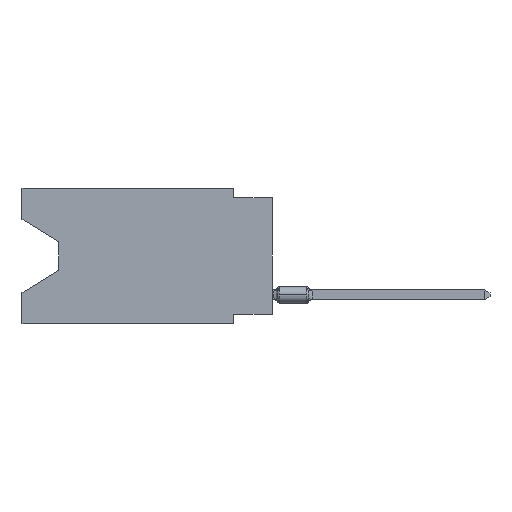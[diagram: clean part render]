
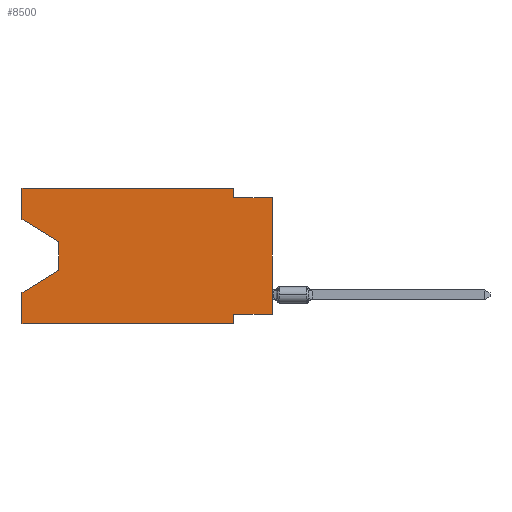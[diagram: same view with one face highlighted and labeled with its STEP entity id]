
A CAD part, left-side view. The second image highlights one B-rep face of the part: STEP entity #8500.
In plain terms, the highlighted planar face has unit normal (-1, 0, 0).
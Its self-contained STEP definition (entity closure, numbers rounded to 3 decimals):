
#78 = CARTESIAN_POINT ( 'NONE',  ( 0., 16.383, 0. ) ) ;
#345 = VERTEX_POINT ( 'NONE', #19564 ) ;
#853 = VERTEX_POINT ( 'NONE', #15511 ) ;
#1800 = EDGE_LOOP ( 'NONE', ( #27748, #20072, #8516, #16104, #6774, #10300, #17275, #5367, #20971, #21598, #28612, #13708 ) ) ;
#1977 = DIRECTION ( 'NONE',  ( 0., 0., -1. ) ) ;
#2008 = VECTOR ( 'NONE', #23691, 1000. ) ;
#3251 = VECTOR ( 'NONE', #20385, 1000. ) ;
#3297 = AXIS2_PLACEMENT_3D ( 'NONE', #5024, #9683, #28205 ) ;
#3729 = LINE ( 'NONE', #27179, #3251 ) ;
#4278 = CARTESIAN_POINT ( 'NONE',  ( 0., 2.54, -8.89 ) ) ;
#4324 = EDGE_CURVE ( 'NONE', #12260, #11319, #3729, .T. ) ;
#4360 = VERTEX_POINT ( 'NONE', #15780 ) ;
#4944 = DIRECTION ( 'NONE',  ( 0., 1., 0. ) ) ;
#5024 = CARTESIAN_POINT ( 'NONE',  ( 0., 16.383, 0. ) ) ;
#5367 = ORIENTED_EDGE ( 'NONE', *, *, #4324, .T. ) ;
#5720 = DIRECTION ( 'NONE',  ( 0., 0., -1. ) ) ;
#6063 = EDGE_CURVE ( 'NONE', #16725, #4360, #11096, .T. ) ;
#6774 = ORIENTED_EDGE ( 'NONE', *, *, #14630, .T. ) ;
#8034 = CARTESIAN_POINT ( 'NONE',  ( 0., 2.54, -8.255 ) ) ;
#8378 = CARTESIAN_POINT ( 'NONE',  ( 0., 0., -0.635 ) ) ;
#8500 = ADVANCED_FACE ( 'NONE', ( #30499 ), #18948, .F. ) ;
#8516 = ORIENTED_EDGE ( 'NONE', *, *, #21570, .T. ) ;
#8838 = VECTOR ( 'NONE', #27270, 1000. ) ;
#8897 = VERTEX_POINT ( 'NONE', #9176 ) ;
#8910 = EDGE_CURVE ( 'NONE', #28071, #29091, #14291, .T. ) ;
#8957 = LINE ( 'NONE', #27643, #15032 ) ;
#9023 = CARTESIAN_POINT ( 'NONE',  ( 0., 16.383, 0. ) ) ;
#9114 = EDGE_CURVE ( 'NONE', #345, #11319, #13198, .T. ) ;
#9176 = CARTESIAN_POINT ( 'NONE',  ( 0., 16.383, -6.852 ) ) ;
#9683 = DIRECTION ( 'NONE',  ( 1., 0., 0. ) ) ;
#10146 = EDGE_CURVE ( 'NONE', #12260, #16725, #20871, .T. ) ;
#10167 = LINE ( 'NONE', #19584, #15781 ) ;
#10300 = ORIENTED_EDGE ( 'NONE', *, *, #6063, .F. ) ;
#10469 = VECTOR ( 'NONE', #5720, 1000. ) ;
#10510 = CARTESIAN_POINT ( 'NONE',  ( 0., 13.97, -3.505 ) ) ;
#10679 = DIRECTION ( 'NONE',  ( 0., 0., -1. ) ) ;
#11096 = LINE ( 'NONE', #4278, #27362 ) ;
#11319 = VERTEX_POINT ( 'NONE', #28081 ) ;
#12260 = VERTEX_POINT ( 'NONE', #25673 ) ;
#12790 = LINE ( 'NONE', #18027, #8838 ) ;
#12844 = VECTOR ( 'NONE', #20445, 1000. ) ;
#12995 = LINE ( 'NONE', #10510, #14455 ) ;
#13198 = LINE ( 'NONE', #8378, #22211 ) ;
#13708 = ORIENTED_EDGE ( 'NONE', *, *, #8910, .F. ) ;
#13918 = CARTESIAN_POINT ( 'NONE',  ( 0., 13.97, -5.385 ) ) ;
#14291 = LINE ( 'NONE', #78, #2008 ) ;
#14455 = VECTOR ( 'NONE', #10679, 1000. ) ;
#14630 = EDGE_CURVE ( 'NONE', #15749, #4360, #10167, .T. ) ;
#14807 = VECTOR ( 'NONE', #4944, 1000. ) ;
#14820 = EDGE_CURVE ( 'NONE', #15749, #8897, #12790, .T. ) ;
#14952 = VECTOR ( 'NONE', #22784, 1000. ) ;
#15032 = VECTOR ( 'NONE', #29961, 1000. ) ;
#15265 = EDGE_CURVE ( 'NONE', #28071, #853, #26936, .T. ) ;
#15511 = CARTESIAN_POINT ( 'NONE',  ( 0., 13.97, -3.505 ) ) ;
#15749 = VERTEX_POINT ( 'NONE', #22546 ) ;
#15780 = CARTESIAN_POINT ( 'NONE',  ( 0., 2.54, -8.89 ) ) ;
#15781 = VECTOR ( 'NONE', #28996, 1000. ) ;
#16104 = ORIENTED_EDGE ( 'NONE', *, *, #14820, .F. ) ;
#16142 = CARTESIAN_POINT ( 'NONE',  ( 0., 16.383, 0. ) ) ;
#16725 = VERTEX_POINT ( 'NONE', #8034 ) ;
#17275 = ORIENTED_EDGE ( 'NONE', *, *, #10146, .F. ) ;
#17475 = CARTESIAN_POINT ( 'NONE',  ( 0., 2.54, 0. ) ) ;
#18027 = CARTESIAN_POINT ( 'NONE',  ( 0., 16.383, 0. ) ) ;
#18045 = VERTEX_POINT ( 'NONE', #24868 ) ;
#18857 = CARTESIAN_POINT ( 'NONE',  ( 0., 0., -8.255 ) ) ;
#18948 = PLANE ( 'NONE',  #3297 ) ;
#19516 = EDGE_CURVE ( 'NONE', #29091, #18045, #30167, .T. ) ;
#19564 = CARTESIAN_POINT ( 'NONE',  ( 0., 2.54, -0.635 ) ) ;
#19584 = CARTESIAN_POINT ( 'NONE',  ( 0., 16.383, -8.89 ) ) ;
#19981 = DIRECTION ( 'NONE',  ( 0., -1., 0. ) ) ;
#20072 = ORIENTED_EDGE ( 'NONE', *, *, #29893, .T. ) ;
#20385 = DIRECTION ( 'NONE',  ( 0., 0., 1. ) ) ;
#20445 = DIRECTION ( 'NONE',  ( 0., -0.855, -0.519 ) ) ;
#20871 = LINE ( 'NONE', #18857, #14807 ) ;
#20971 = ORIENTED_EDGE ( 'NONE', *, *, #9114, .F. ) ;
#21570 = EDGE_CURVE ( 'NONE', #30261, #8897, #8957, .T. ) ;
#21598 = ORIENTED_EDGE ( 'NONE', *, *, #29772, .F. ) ;
#22211 = VECTOR ( 'NONE', #19981, 1000. ) ;
#22546 = CARTESIAN_POINT ( 'NONE',  ( 0., 16.383, -8.89 ) ) ;
#22784 = DIRECTION ( 'NONE',  ( 0., -1., 0. ) ) ;
#23691 = DIRECTION ( 'NONE',  ( 0., 0., 1. ) ) ;
#23962 = LINE ( 'NONE', #17475, #10469 ) ;
#24868 = CARTESIAN_POINT ( 'NONE',  ( 0., 2.54, 0. ) ) ;
#25673 = CARTESIAN_POINT ( 'NONE',  ( 0., 0., -8.255 ) ) ;
#26936 = LINE ( 'NONE', #29245, #12844 ) ;
#27179 = CARTESIAN_POINT ( 'NONE',  ( 0., 0., 0. ) ) ;
#27270 = DIRECTION ( 'NONE',  ( 0., 0., 1. ) ) ;
#27362 = VECTOR ( 'NONE', #1977, 1000. ) ;
#27643 = CARTESIAN_POINT ( 'NONE',  ( 0., 13.97, -5.385 ) ) ;
#27748 = ORIENTED_EDGE ( 'NONE', *, *, #15265, .T. ) ;
#28071 = VERTEX_POINT ( 'NONE', #29216 ) ;
#28081 = CARTESIAN_POINT ( 'NONE',  ( 0., 0., -0.635 ) ) ;
#28205 = DIRECTION ( 'NONE',  ( 0., 0., -1. ) ) ;
#28612 = ORIENTED_EDGE ( 'NONE', *, *, #19516, .F. ) ;
#28996 = DIRECTION ( 'NONE',  ( 0., -1., 0. ) ) ;
#29091 = VERTEX_POINT ( 'NONE', #16142 ) ;
#29216 = CARTESIAN_POINT ( 'NONE',  ( 0., 16.383, -2.038 ) ) ;
#29245 = CARTESIAN_POINT ( 'NONE',  ( 0., 16.383, -2.038 ) ) ;
#29772 = EDGE_CURVE ( 'NONE', #18045, #345, #23962, .T. ) ;
#29893 = EDGE_CURVE ( 'NONE', #853, #30261, #12995, .T. ) ;
#29961 = DIRECTION ( 'NONE',  ( 0., 0.855, -0.519 ) ) ;
#30167 = LINE ( 'NONE', #9023, #14952 ) ;
#30261 = VERTEX_POINT ( 'NONE', #13918 ) ;
#30499 = FACE_OUTER_BOUND ( 'NONE', #1800, .T. ) ;
